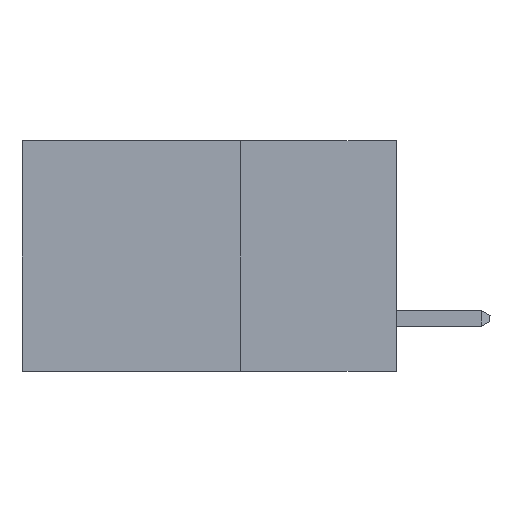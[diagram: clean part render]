
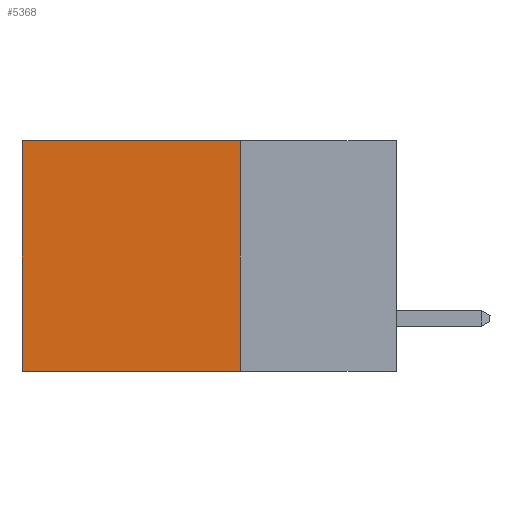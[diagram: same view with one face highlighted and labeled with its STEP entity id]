
A CAD part, left-side view. The second image highlights one B-rep face of the part: STEP entity #5368.
In plain terms, the highlighted planar face has unit normal (-1, 0, 0).
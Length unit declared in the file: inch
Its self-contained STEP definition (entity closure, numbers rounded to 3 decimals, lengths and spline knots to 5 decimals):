
#674 = CARTESIAN_POINT ( 'NONE',  ( 0.2615, 0.25, -0.37 ) ) ;
#2308 = LINE ( 'NONE', #10274, #14557 ) ;
#3071 = VECTOR ( 'NONE', #15009, 39.37008 ) ;
#3291 = VERTEX_POINT ( 'NONE', #12201 ) ;
#4227 = DIRECTION ( 'NONE',  ( 0., 0., -1. ) ) ;
#4290 = DIRECTION ( 'NONE',  ( 0., 0., -1. ) ) ;
#4399 = ORIENTED_EDGE ( 'NONE', *, *, #5116, .F. ) ;
#4660 = EDGE_CURVE ( 'NONE', #9333, #6446, #14969, .T. ) ;
#5116 = EDGE_CURVE ( 'NONE', #14762, #6446, #16460, .T. ) ;
#5368 = ADVANCED_FACE ( 'NONE', ( #9504 ), #13268, .F. ) ;
#6070 = EDGE_CURVE ( 'NONE', #3291, #14762, #2308, .T. ) ;
#6198 = DIRECTION ( 'NONE',  ( 0., 1., 0. ) ) ;
#6446 = VERTEX_POINT ( 'NONE', #14023 ) ;
#6712 = VECTOR ( 'NONE', #6198, 39.37008 ) ;
#8518 = ORIENTED_EDGE ( 'NONE', *, *, #15330, .T. ) ;
#8878 = LINE ( 'NONE', #11712, #6712 ) ;
#9333 = VERTEX_POINT ( 'NONE', #14988 ) ;
#9504 = FACE_OUTER_BOUND ( 'NONE', #9626, .T. ) ;
#9626 = EDGE_LOOP ( 'NONE', ( #11003, #4399, #12800, #8518 ) ) ;
#9776 = CARTESIAN_POINT ( 'NONE',  ( 0.2615, 0.25, -0.37 ) ) ;
#10274 = CARTESIAN_POINT ( 'NONE',  ( 0.2615, 0.25, -0.37 ) ) ;
#10614 = CARTESIAN_POINT ( 'NONE',  ( 0.2615, 0.25, -0.37 ) ) ;
#11003 = ORIENTED_EDGE ( 'NONE', *, *, #4660, .T. ) ;
#11712 = CARTESIAN_POINT ( 'NONE',  ( 0.2615, 0.25, 0. ) ) ;
#11805 = DIRECTION ( 'NONE',  ( 0., 0., -1. ) ) ;
#11990 = DIRECTION ( 'NONE',  ( 1., 0., 0. ) ) ;
#12201 = CARTESIAN_POINT ( 'NONE',  ( 0.2615, 0.25, 0. ) ) ;
#12330 = AXIS2_PLACEMENT_3D ( 'NONE', #10614, #11990, #4227 ) ;
#12800 = ORIENTED_EDGE ( 'NONE', *, *, #6070, .F. ) ;
#13268 = PLANE ( 'NONE',  #12330 ) ;
#13602 = VECTOR ( 'NONE', #4290, 39.37008 ) ;
#14023 = CARTESIAN_POINT ( 'NONE',  ( 0.2615, 0.6, -0.37 ) ) ;
#14557 = VECTOR ( 'NONE', #11805, 39.37008 ) ;
#14762 = VERTEX_POINT ( 'NONE', #674 ) ;
#14890 = CARTESIAN_POINT ( 'NONE',  ( 0.2615, 0.6, -0.37 ) ) ;
#14969 = LINE ( 'NONE', #14890, #13602 ) ;
#14988 = CARTESIAN_POINT ( 'NONE',  ( 0.2615, 0.6, 0. ) ) ;
#15009 = DIRECTION ( 'NONE',  ( 0., 1., 0. ) ) ;
#15330 = EDGE_CURVE ( 'NONE', #3291, #9333, #8878, .T. ) ;
#16460 = LINE ( 'NONE', #9776, #3071 ) ;
